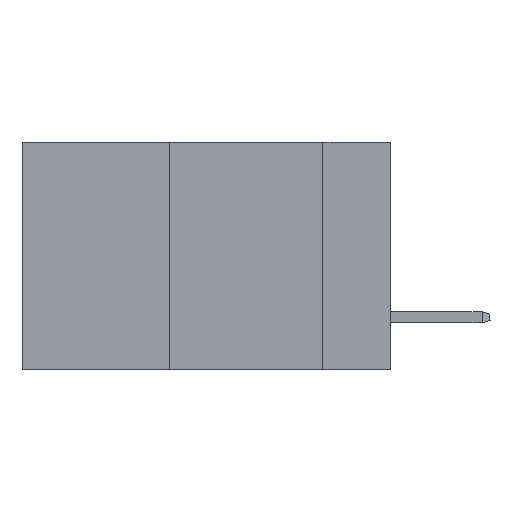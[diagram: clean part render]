
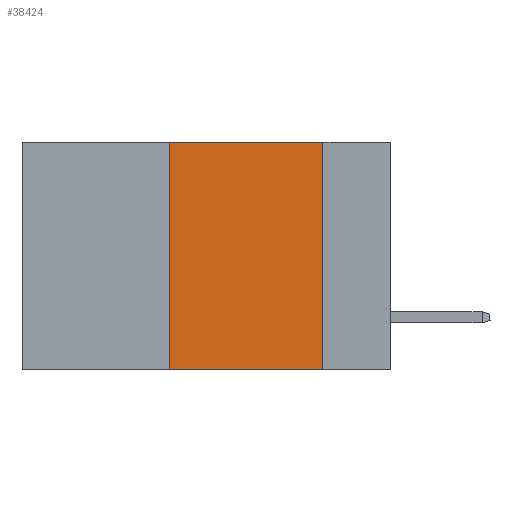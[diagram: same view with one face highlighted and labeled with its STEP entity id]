
A CAD part, left-side view. The second image highlights one B-rep face of the part: STEP entity #38424.
In plain terms, the highlighted planar face has unit normal (-1, 0, 0).
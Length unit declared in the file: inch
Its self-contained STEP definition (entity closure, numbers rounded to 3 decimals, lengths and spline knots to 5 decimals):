
#602 = EDGE_CURVE ( 'NONE', #23117, #12811, #5084, .T. ) ;
#914 = DIRECTION ( 'NONE',  ( 0., 0., -1. ) ) ;
#2927 = ORIENTED_EDGE ( 'NONE', *, *, #38735, .F. ) ;
#3530 = VECTOR ( 'NONE', #37034, 39.37008 ) ;
#3863 = AXIS2_PLACEMENT_3D ( 'NONE', #22977, #29516, #914 ) ;
#5084 = LINE ( 'NONE', #35856, #25889 ) ;
#6805 = CARTESIAN_POINT ( 'NONE',  ( 0., 0.11, -0.37 ) ) ;
#9572 = DIRECTION ( 'NONE',  ( 0., 0., 1. ) ) ;
#12811 = VERTEX_POINT ( 'NONE', #6805 ) ;
#13740 = EDGE_CURVE ( 'NONE', #33316, #12811, #29311, .T. ) ;
#14190 = DIRECTION ( 'NONE',  ( 0., -1., 0. ) ) ;
#14505 = CARTESIAN_POINT ( 'NONE',  ( 0., 0.6, 0. ) ) ;
#14784 = CARTESIAN_POINT ( 'NONE',  ( 0., 0.11, 0. ) ) ;
#18880 = CARTESIAN_POINT ( 'NONE',  ( 0., 0.11, 0. ) ) ;
#20208 = ORIENTED_EDGE ( 'NONE', *, *, #13740, .F. ) ;
#20222 = PLANE ( 'NONE',  #3863 ) ;
#20388 = LINE ( 'NONE', #22186, #22399 ) ;
#21247 = CARTESIAN_POINT ( 'NONE',  ( 0., 0.36, 0. ) ) ;
#21467 = VECTOR ( 'NONE', #26970, 39.37008 ) ;
#22186 = CARTESIAN_POINT ( 'NONE',  ( 0., 0.36, 0. ) ) ;
#22399 = VECTOR ( 'NONE', #9572, 39.37008 ) ;
#22411 = LINE ( 'NONE', #14505, #21467 ) ;
#22492 = EDGE_LOOP ( 'NONE', ( #20208, #35479, #2927, #40036 ) ) ;
#22977 = CARTESIAN_POINT ( 'NONE',  ( 0., 0.6, 0. ) ) ;
#23117 = VERTEX_POINT ( 'NONE', #34401 ) ;
#23484 = EDGE_CURVE ( 'NONE', #41058, #33316, #22411, .T. ) ;
#25889 = VECTOR ( 'NONE', #14190, 39.37008 ) ;
#26970 = DIRECTION ( 'NONE',  ( 0., -1., 0. ) ) ;
#29311 = LINE ( 'NONE', #14784, #3530 ) ;
#29516 = DIRECTION ( 'NONE',  ( 1., 0., 0. ) ) ;
#33316 = VERTEX_POINT ( 'NONE', #18880 ) ;
#34401 = CARTESIAN_POINT ( 'NONE',  ( 0., 0.36, -0.37 ) ) ;
#35479 = ORIENTED_EDGE ( 'NONE', *, *, #23484, .F. ) ;
#35856 = CARTESIAN_POINT ( 'NONE',  ( 0., 0.6, -0.37 ) ) ;
#37034 = DIRECTION ( 'NONE',  ( 0., 0., -1. ) ) ;
#38424 = ADVANCED_FACE ( 'NONE', ( #38768 ), #20222, .F. ) ;
#38735 = EDGE_CURVE ( 'NONE', #23117, #41058, #20388, .T. ) ;
#38768 = FACE_OUTER_BOUND ( 'NONE', #22492, .T. ) ;
#40036 = ORIENTED_EDGE ( 'NONE', *, *, #602, .T. ) ;
#41058 = VERTEX_POINT ( 'NONE', #21247 ) ;
